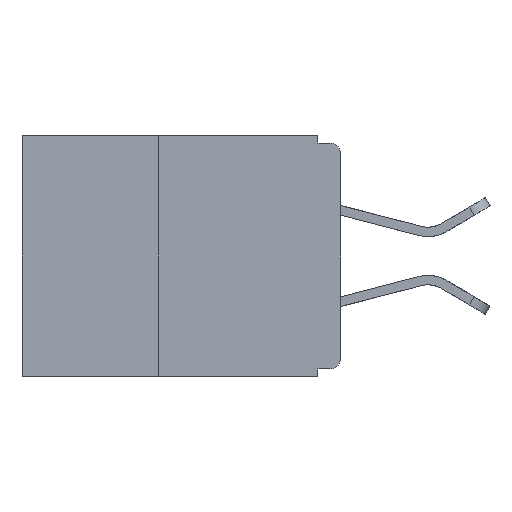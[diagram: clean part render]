
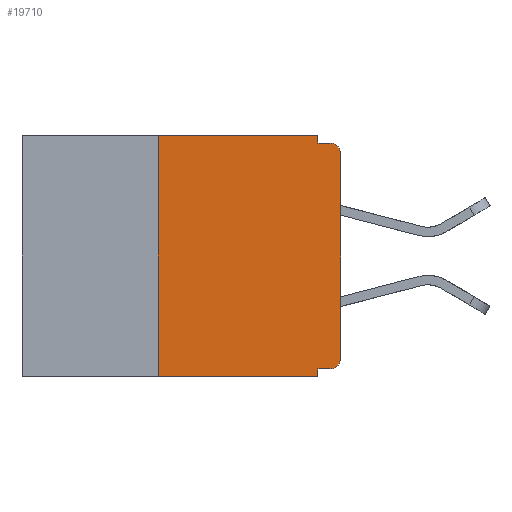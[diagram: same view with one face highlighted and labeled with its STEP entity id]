
A CAD part, left-side view. The second image highlights one B-rep face of the part: STEP entity #19710.
In plain terms, the highlighted planar face has unit normal (-1, 0, 0).
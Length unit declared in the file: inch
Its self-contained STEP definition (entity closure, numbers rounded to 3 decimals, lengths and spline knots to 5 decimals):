
#136 = LINE ( 'NONE', #4575, #6680 ) ;
#724 = AXIS2_PLACEMENT_3D ( 'NONE', #7817, #24603, #10234 ) ;
#801 = LINE ( 'NONE', #21868, #20843 ) ;
#1216 = VERTEX_POINT ( 'NONE', #25607 ) ;
#1394 = DIRECTION ( 'NONE',  ( 0., 0., -1. ) ) ;
#1462 = DIRECTION ( 'NONE',  ( -1., 0., 0. ) ) ;
#1545 = CARTESIAN_POINT ( 'NONE',  ( 0., 0.25, -0.33 ) ) ;
#1652 = VERTEX_POINT ( 'NONE', #29838 ) ;
#1664 = CARTESIAN_POINT ( 'NONE',  ( 0., 0.031, -0.32 ) ) ;
#1673 = CARTESIAN_POINT ( 'NONE',  ( 0., 0.015, -0.305 ) ) ;
#2907 = FACE_OUTER_BOUND ( 'NONE', #14835, .T. ) ;
#2911 = VECTOR ( 'NONE', #8110, 39.37008 ) ;
#3187 = ORIENTED_EDGE ( 'NONE', *, *, #16336, .T. ) ;
#3317 = ORIENTED_EDGE ( 'NONE', *, *, #16017, .F. ) ;
#3601 = EDGE_CURVE ( 'NONE', #25981, #11253, #27488, .T. ) ;
#3884 = EDGE_CURVE ( 'NONE', #17980, #14729, #801, .T. ) ;
#4142 = CARTESIAN_POINT ( 'NONE',  ( 0., 0.031, -0.01 ) ) ;
#4286 = CARTESIAN_POINT ( 'NONE',  ( 0., 0.25, 0. ) ) ;
#4575 = CARTESIAN_POINT ( 'NONE',  ( 0., 0.031, 0. ) ) ;
#4914 = VERTEX_POINT ( 'NONE', #1664 ) ;
#5225 = PLANE ( 'NONE',  #23090 ) ;
#6482 = AXIS2_PLACEMENT_3D ( 'NONE', #1673, #1462, #1394 ) ;
#6680 = VECTOR ( 'NONE', #30743, 39.37008 ) ;
#7642 = DIRECTION ( 'NONE',  ( 0., 0., -1. ) ) ;
#7817 = CARTESIAN_POINT ( 'NONE',  ( 0., 0.015, -0.025 ) ) ;
#8110 = DIRECTION ( 'NONE',  ( 0., -1., 0. ) ) ;
#8516 = EDGE_CURVE ( 'NONE', #25981, #4914, #29211, .T. ) ;
#8706 = VECTOR ( 'NONE', #16010, 39.37008 ) ;
#8754 = VECTOR ( 'NONE', #10810, 39.37008 ) ;
#8835 = ORIENTED_EDGE ( 'NONE', *, *, #28015, .F. ) ;
#9363 = LINE ( 'NONE', #27123, #2911 ) ;
#10234 = DIRECTION ( 'NONE',  ( 0., 0., -1. ) ) ;
#10544 = LINE ( 'NONE', #20772, #28057 ) ;
#10810 = DIRECTION ( 'NONE',  ( 0., 1., 0. ) ) ;
#11253 = VERTEX_POINT ( 'NONE', #13780 ) ;
#12108 = ORIENTED_EDGE ( 'NONE', *, *, #23953, .F. ) ;
#12216 = ORIENTED_EDGE ( 'NONE', *, *, #8516, .F. ) ;
#12484 = VERTEX_POINT ( 'NONE', #4286 ) ;
#12504 = DIRECTION ( 'NONE',  ( 0., -1., 0. ) ) ;
#12867 = CARTESIAN_POINT ( 'NONE',  ( 0., 0.25, -0.33 ) ) ;
#13780 = CARTESIAN_POINT ( 'NONE',  ( 0., 0., -0.305 ) ) ;
#14729 = VERTEX_POINT ( 'NONE', #17495 ) ;
#14835 = EDGE_LOOP ( 'NONE', ( #3187, #20663, #24227, #8835, #23125, #12108, #20588, #3317, #12216, #22592 ) ) ;
#15090 = LINE ( 'NONE', #1545, #8706 ) ;
#15221 = EDGE_CURVE ( 'NONE', #17273, #14729, #16354, .T. ) ;
#15907 = VECTOR ( 'NONE', #16749, 39.37008 ) ;
#16010 = DIRECTION ( 'NONE',  ( 0., 0., 1. ) ) ;
#16017 = EDGE_CURVE ( 'NONE', #4914, #1216, #30303, .T. ) ;
#16336 = EDGE_CURVE ( 'NONE', #11253, #17273, #23057, .T. ) ;
#16354 = CIRCLE ( 'NONE', #724, 0.015 ) ;
#16749 = DIRECTION ( 'NONE',  ( 0., 0., 1. ) ) ;
#17187 = CARTESIAN_POINT ( 'NONE',  ( 0., 0.437, 0. ) ) ;
#17273 = VERTEX_POINT ( 'NONE', #20621 ) ;
#17495 = CARTESIAN_POINT ( 'NONE',  ( 0., 0.015, -0.01 ) ) ;
#17803 = VECTOR ( 'NONE', #20357, 39.37008 ) ;
#17934 = CARTESIAN_POINT ( 'NONE',  ( 0., 0.031, -0.33 ) ) ;
#17957 = EDGE_CURVE ( 'NONE', #12484, #1652, #10544, .T. ) ;
#17980 = VERTEX_POINT ( 'NONE', #4142 ) ;
#18469 = DIRECTION ( 'NONE',  ( 0., -1., 0. ) ) ;
#18626 = EDGE_CURVE ( 'NONE', #26549, #1216, #9363, .T. ) ;
#19710 = ADVANCED_FACE ( 'NONE', ( #2907 ), #5225, .F. ) ;
#20357 = DIRECTION ( 'NONE',  ( 0., 0., -1. ) ) ;
#20588 = ORIENTED_EDGE ( 'NONE', *, *, #18626, .T. ) ;
#20621 = CARTESIAN_POINT ( 'NONE',  ( 0., 0., -0.025 ) ) ;
#20663 = ORIENTED_EDGE ( 'NONE', *, *, #15221, .T. ) ;
#20772 = CARTESIAN_POINT ( 'NONE',  ( 0., 0.437, 0. ) ) ;
#20843 = VECTOR ( 'NONE', #12504, 39.37008 ) ;
#21868 = CARTESIAN_POINT ( 'NONE',  ( 0., 0., -0.01 ) ) ;
#22039 = DIRECTION ( 'NONE',  ( 1., 0., 0. ) ) ;
#22459 = CARTESIAN_POINT ( 'NONE',  ( 0., 0.015, -0.32 ) ) ;
#22592 = ORIENTED_EDGE ( 'NONE', *, *, #3601, .T. ) ;
#23057 = LINE ( 'NONE', #26127, #15907 ) ;
#23090 = AXIS2_PLACEMENT_3D ( 'NONE', #17187, #22039, #7642 ) ;
#23125 = ORIENTED_EDGE ( 'NONE', *, *, #17957, .F. ) ;
#23953 = EDGE_CURVE ( 'NONE', #26549, #12484, #15090, .T. ) ;
#24227 = ORIENTED_EDGE ( 'NONE', *, *, #3884, .F. ) ;
#24603 = DIRECTION ( 'NONE',  ( -1., 0., 0. ) ) ;
#25052 = CARTESIAN_POINT ( 'NONE',  ( 0., 0., -0.32 ) ) ;
#25607 = CARTESIAN_POINT ( 'NONE',  ( 0., 0.031, -0.33 ) ) ;
#25981 = VERTEX_POINT ( 'NONE', #22459 ) ;
#26127 = CARTESIAN_POINT ( 'NONE',  ( 0., 0., 0. ) ) ;
#26549 = VERTEX_POINT ( 'NONE', #12867 ) ;
#27123 = CARTESIAN_POINT ( 'NONE',  ( 0., 0.437, -0.33 ) ) ;
#27488 = CIRCLE ( 'NONE', #6482, 0.015 ) ;
#28015 = EDGE_CURVE ( 'NONE', #1652, #17980, #136, .T. ) ;
#28057 = VECTOR ( 'NONE', #18469, 39.37008 ) ;
#29211 = LINE ( 'NONE', #25052, #8754 ) ;
#29838 = CARTESIAN_POINT ( 'NONE',  ( 0., 0.031, 0. ) ) ;
#30303 = LINE ( 'NONE', #17934, #17803 ) ;
#30743 = DIRECTION ( 'NONE',  ( 0., 0., -1. ) ) ;
